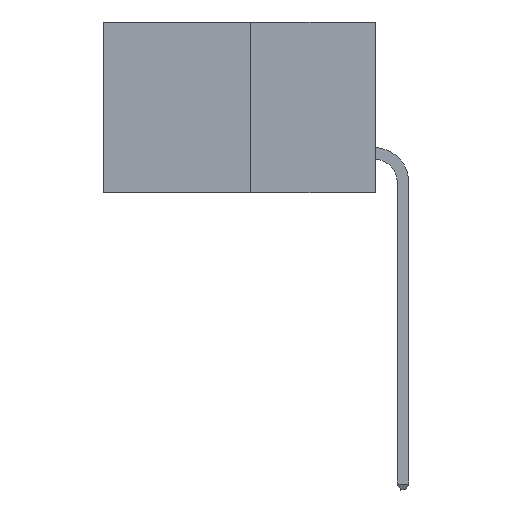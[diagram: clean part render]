
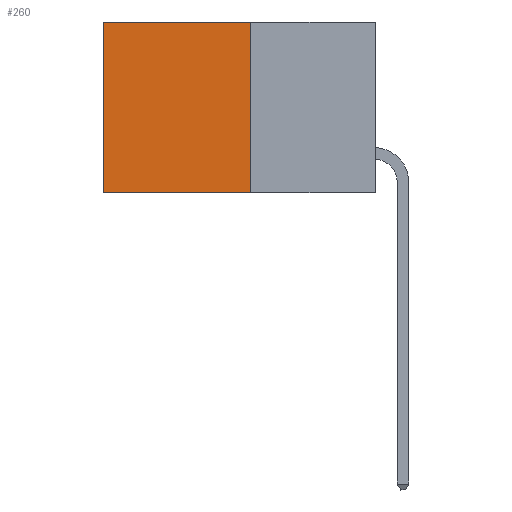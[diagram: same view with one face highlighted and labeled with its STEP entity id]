
A CAD part, left-side view. The second image highlights one B-rep face of the part: STEP entity #260.
In plain terms, the highlighted planar face has unit normal (-1, 0, 0).
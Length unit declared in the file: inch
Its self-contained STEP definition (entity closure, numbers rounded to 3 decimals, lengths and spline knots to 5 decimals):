
#169 = CARTESIAN_POINT ( 'NONE',  ( 0.277, 0.27, -0.37 ) ) ;
#260 = ADVANCED_FACE ( 'NONE', ( #6322 ), #6460, .F. ) ;
#312 = EDGE_CURVE ( 'NONE', #1043, #2273, #7291, .T. ) ;
#422 = VECTOR ( 'NONE', #2270, 39.37008 ) ;
#437 = EDGE_CURVE ( 'NONE', #2554, #2807, #1009, .T. ) ;
#641 = EDGE_LOOP ( 'NONE', ( #1917, #3219, #2126, #4408 ) ) ;
#1009 = LINE ( 'NONE', #6153, #4529 ) ;
#1043 = VERTEX_POINT ( 'NONE', #2432 ) ;
#1390 = CARTESIAN_POINT ( 'NONE',  ( 0.277, 0.59, 0. ) ) ;
#1647 = CARTESIAN_POINT ( 'NONE',  ( 0.277, 0.59, -0.37 ) ) ;
#1778 = DIRECTION ( 'NONE',  ( 0., 0., -1. ) ) ;
#1917 = ORIENTED_EDGE ( 'NONE', *, *, #6584, .T. ) ;
#2116 = DIRECTION ( 'NONE',  ( 0., 1., 0. ) ) ;
#2126 = ORIENTED_EDGE ( 'NONE', *, *, #6163, .F. ) ;
#2260 = DIRECTION ( 'NONE',  ( 0., 0., -1. ) ) ;
#2270 = DIRECTION ( 'NONE',  ( 0., 1., 0. ) ) ;
#2273 = VERTEX_POINT ( 'NONE', #1390 ) ;
#2432 = CARTESIAN_POINT ( 'NONE',  ( 0.277, 0.27, 0. ) ) ;
#2554 = VERTEX_POINT ( 'NONE', #169 ) ;
#2807 = VERTEX_POINT ( 'NONE', #3001 ) ;
#3001 = CARTESIAN_POINT ( 'NONE',  ( 0.277, 0.59, -0.37 ) ) ;
#3219 = ORIENTED_EDGE ( 'NONE', *, *, #437, .F. ) ;
#3407 = AXIS2_PLACEMENT_3D ( 'NONE', #7959, #3535, #3446 ) ;
#3446 = DIRECTION ( 'NONE',  ( 0., 0., -1. ) ) ;
#3535 = DIRECTION ( 'NONE',  ( 1., 0., 0. ) ) ;
#4408 = ORIENTED_EDGE ( 'NONE', *, *, #312, .T. ) ;
#4529 = VECTOR ( 'NONE', #2116, 39.37008 ) ;
#4539 = VECTOR ( 'NONE', #2260, 39.37008 ) ;
#4558 = CARTESIAN_POINT ( 'NONE',  ( 0.277, 0.27, 0. ) ) ;
#4645 = LINE ( 'NONE', #1647, #7843 ) ;
#4740 = LINE ( 'NONE', #5681, #4539 ) ;
#5681 = CARTESIAN_POINT ( 'NONE',  ( 0.277, 0.27, -0.37 ) ) ;
#6153 = CARTESIAN_POINT ( 'NONE',  ( 0.277, 0.27, -0.37 ) ) ;
#6163 = EDGE_CURVE ( 'NONE', #1043, #2554, #4740, .T. ) ;
#6322 = FACE_OUTER_BOUND ( 'NONE', #641, .T. ) ;
#6460 = PLANE ( 'NONE',  #3407 ) ;
#6584 = EDGE_CURVE ( 'NONE', #2273, #2807, #4645, .T. ) ;
#7291 = LINE ( 'NONE', #4558, #422 ) ;
#7843 = VECTOR ( 'NONE', #1778, 39.37008 ) ;
#7959 = CARTESIAN_POINT ( 'NONE',  ( 0.277, 0.27, -0.37 ) ) ;
